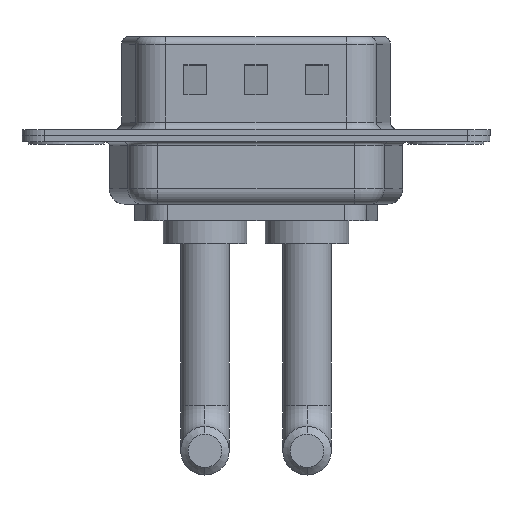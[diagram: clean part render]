
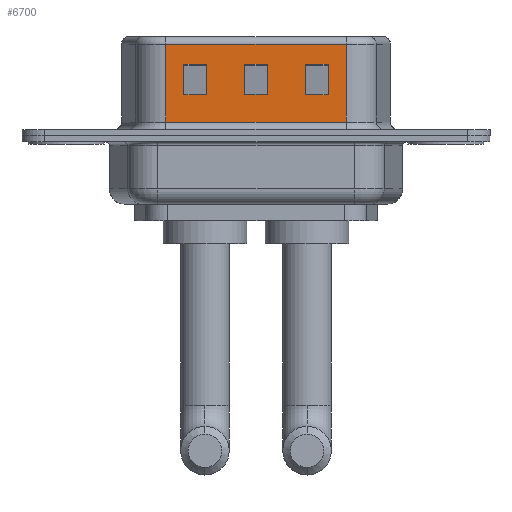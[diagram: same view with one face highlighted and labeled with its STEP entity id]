
A CAD part, front view. The second image highlights one B-rep face of the part: STEP entity #6700.
In plain terms, the highlighted planar face has unit normal (0, -1, 0).
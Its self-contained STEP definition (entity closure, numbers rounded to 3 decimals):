
#127 = EDGE_CURVE ( 'NONE', #7532, #10538, #2678, .T. ) ;
#140 = LINE ( 'NONE', #11574, #12310 ) ;
#228 = ORIENTED_EDGE ( 'NONE', *, *, #10622, .T. ) ;
#281 = DIRECTION ( 'NONE',  ( 0., 0., 1. ) ) ;
#351 = LINE ( 'NONE', #2179, #9631 ) ;
#443 = VERTEX_POINT ( 'NONE', #8490 ) ;
#605 = CARTESIAN_POINT ( 'NONE',  ( 18.451, -4.55, 0.9 ) ) ;
#623 = DIRECTION ( 'NONE',  ( 0., 1., 0. ) ) ;
#630 = CARTESIAN_POINT ( 'NONE',  ( 6.549, -4.55, 6.02 ) ) ;
#771 = ORIENTED_EDGE ( 'NONE', *, *, #10934, .F. ) ;
#1061 = ORIENTED_EDGE ( 'NONE', *, *, #8259, .T. ) ;
#1787 = EDGE_LOOP ( 'NONE', ( #228, #11066, #6406, #2359 ) ) ;
#1797 = FACE_BOUND ( 'NONE', #4188, .T. ) ;
#1937 = DIRECTION ( 'NONE',  ( 0., 0., -1. ) ) ;
#2086 = LINE ( 'NONE', #3164, #5693 ) ;
#2090 = CARTESIAN_POINT ( 'NONE',  ( 18.451, -4.55, 6.02 ) ) ;
#2119 = VECTOR ( 'NONE', #6483, 1000. ) ;
#2145 = DIRECTION ( 'NONE',  ( 1., 0., 0. ) ) ;
#2179 = CARTESIAN_POINT ( 'NONE',  ( 15.75, -4.55, 6.52 ) ) ;
#2353 = VERTEX_POINT ( 'NONE', #2929 ) ;
#2359 = ORIENTED_EDGE ( 'NONE', *, *, #7183, .T. ) ;
#2406 = LINE ( 'NONE', #5481, #9683 ) ;
#2586 = LINE ( 'NONE', #6353, #2119 ) ;
#2648 = EDGE_LOOP ( 'NONE', ( #1061, #12330, #9384, #11401 ) ) ;
#2678 = LINE ( 'NONE', #8633, #5533 ) ;
#2910 = DIRECTION ( 'NONE',  ( 1., 0., 0. ) ) ;
#2929 = CARTESIAN_POINT ( 'NONE',  ( 17.25, -4.55, 2.705 ) ) ;
#2930 = EDGE_CURVE ( 'NONE', #5158, #11398, #2086, .T. ) ;
#3065 = EDGE_CURVE ( 'NONE', #11744, #443, #2406, .T. ) ;
#3164 = CARTESIAN_POINT ( 'NONE',  ( 18.451, -4.55, 2.705 ) ) ;
#3402 = ORIENTED_EDGE ( 'NONE', *, *, #8332, .T. ) ;
#3432 = CARTESIAN_POINT ( 'NONE',  ( 18.451, -4.55, 6.52 ) ) ;
#3457 = VERTEX_POINT ( 'NONE', #6943 ) ;
#3461 = CARTESIAN_POINT ( 'NONE',  ( 15.75, -4.55, 4.705 ) ) ;
#3590 = CARTESIAN_POINT ( 'NONE',  ( 11.75, -4.55, 2.705 ) ) ;
#3946 = VECTOR ( 'NONE', #10274, 1000. ) ;
#4059 = DIRECTION ( 'NONE',  ( 0., 0., -1. ) ) ;
#4090 = EDGE_CURVE ( 'NONE', #2353, #8831, #5876, .T. ) ;
#4129 = DIRECTION ( 'NONE',  ( 1., 0., 0. ) ) ;
#4188 = EDGE_LOOP ( 'NONE', ( #3402, #8569, #7565, #4711 ) ) ;
#4375 = CARTESIAN_POINT ( 'NONE',  ( 18.451, -4.55, 4.705 ) ) ;
#4378 = VERTEX_POINT ( 'NONE', #6639 ) ;
#4633 = PLANE ( 'NONE',  #5189 ) ;
#4634 = VERTEX_POINT ( 'NONE', #10133 ) ;
#4681 = CARTESIAN_POINT ( 'NONE',  ( 9.25, -4.55, 6.52 ) ) ;
#4711 = ORIENTED_EDGE ( 'NONE', *, *, #9969, .T. ) ;
#4925 = CARTESIAN_POINT ( 'NONE',  ( 9.25, -4.55, 4.705 ) ) ;
#4926 = CARTESIAN_POINT ( 'NONE',  ( 22.451, -4.55, 2.705 ) ) ;
#5158 = VERTEX_POINT ( 'NONE', #11737 ) ;
#5166 = LINE ( 'NONE', #10057, #6983 ) ;
#5189 = AXIS2_PLACEMENT_3D ( 'NONE', #10415, #623, #7556 ) ;
#5291 = DIRECTION ( 'NONE',  ( 0., 0., 1. ) ) ;
#5481 = CARTESIAN_POINT ( 'NONE',  ( 7.75, -4.55, 6.52 ) ) ;
#5533 = VECTOR ( 'NONE', #10711, 1000. ) ;
#5651 = FACE_BOUND ( 'NONE', #1787, .T. ) ;
#5668 = DIRECTION ( 'NONE',  ( 0., 0., 1. ) ) ;
#5693 = VECTOR ( 'NONE', #10802, 1000. ) ;
#5702 = EDGE_CURVE ( 'NONE', #8831, #10414, #351, .T. ) ;
#5755 = VECTOR ( 'NONE', #7916, 1000. ) ;
#5876 = LINE ( 'NONE', #4926, #7566 ) ;
#5933 = CARTESIAN_POINT ( 'NONE',  ( 17.25, -4.55, 4.705 ) ) ;
#6199 = VERTEX_POINT ( 'NONE', #8041 ) ;
#6353 = CARTESIAN_POINT ( 'NONE',  ( 13.25, -4.55, 6.52 ) ) ;
#6406 = ORIENTED_EDGE ( 'NONE', *, *, #5702, .T. ) ;
#6483 = DIRECTION ( 'NONE',  ( 0., 0., -1. ) ) ;
#6567 = CARTESIAN_POINT ( 'NONE',  ( 15.75, -4.55, 2.705 ) ) ;
#6591 = VECTOR ( 'NONE', #5668, 1000. ) ;
#6613 = VECTOR ( 'NONE', #11154, 1000. ) ;
#6639 = CARTESIAN_POINT ( 'NONE',  ( 11.75, -4.55, 4.705 ) ) ;
#6663 = CARTESIAN_POINT ( 'NONE',  ( 17.25, -4.55, 6.52 ) ) ;
#6700 = ADVANCED_FACE ( 'NONE', ( #1797, #5651, #9586, #6711 ), #4633, .F. ) ;
#6711 = FACE_OUTER_BOUND ( 'NONE', #10720, .T. ) ;
#6894 = CARTESIAN_POINT ( 'NONE',  ( 22.451, -4.55, 4.705 ) ) ;
#6943 = CARTESIAN_POINT ( 'NONE',  ( 6.549, -4.55, 0.9 ) ) ;
#6983 = VECTOR ( 'NONE', #4129, 1000. ) ;
#7183 = EDGE_CURVE ( 'NONE', #10414, #7270, #8817, .T. ) ;
#7199 = VECTOR ( 'NONE', #11296, 1000. ) ;
#7270 = VERTEX_POINT ( 'NONE', #5933 ) ;
#7532 = VERTEX_POINT ( 'NONE', #2090 ) ;
#7556 = DIRECTION ( 'NONE',  ( -1., 0., 0. ) ) ;
#7565 = ORIENTED_EDGE ( 'NONE', *, *, #3065, .T. ) ;
#7566 = VECTOR ( 'NONE', #8823, 1000. ) ;
#7599 = VECTOR ( 'NONE', #2910, 1000. ) ;
#7916 = DIRECTION ( 'NONE',  ( 1., 0., 0. ) ) ;
#7946 = LINE ( 'NONE', #4375, #10563 ) ;
#8041 = CARTESIAN_POINT ( 'NONE',  ( 9.25, -4.55, 2.705 ) ) ;
#8066 = LINE ( 'NONE', #11929, #6613 ) ;
#8259 = EDGE_CURVE ( 'NONE', #4378, #4634, #7946, .T. ) ;
#8322 = CARTESIAN_POINT ( 'NONE',  ( 7.75, -4.55, 2.705 ) ) ;
#8332 = EDGE_CURVE ( 'NONE', #11998, #6199, #10349, .T. ) ;
#8434 = LINE ( 'NONE', #3432, #3946 ) ;
#8490 = CARTESIAN_POINT ( 'NONE',  ( 7.75, -4.55, 4.705 ) ) ;
#8538 = LINE ( 'NONE', #8599, #6591 ) ;
#8569 = ORIENTED_EDGE ( 'NONE', *, *, #10892, .T. ) ;
#8599 = CARTESIAN_POINT ( 'NONE',  ( 11.75, -4.55, 6.52 ) ) ;
#8633 = CARTESIAN_POINT ( 'NONE',  ( 18.451, -4.55, 6.02 ) ) ;
#8798 = VERTEX_POINT ( 'NONE', #605 ) ;
#8817 = LINE ( 'NONE', #6894, #5755 ) ;
#8823 = DIRECTION ( 'NONE',  ( -1., 0., 0. ) ) ;
#8831 = VERTEX_POINT ( 'NONE', #6567 ) ;
#9384 = ORIENTED_EDGE ( 'NONE', *, *, #2930, .T. ) ;
#9483 = LINE ( 'NONE', #6663, #11067 ) ;
#9586 = FACE_BOUND ( 'NONE', #2648, .T. ) ;
#9631 = VECTOR ( 'NONE', #281, 1000. ) ;
#9683 = VECTOR ( 'NONE', #5291, 1000. ) ;
#9752 = EDGE_CURVE ( 'NONE', #3457, #8798, #10691, .T. ) ;
#9966 = ORIENTED_EDGE ( 'NONE', *, *, #12376, .T. ) ;
#9969 = EDGE_CURVE ( 'NONE', #443, #11998, #5166, .T. ) ;
#10057 = CARTESIAN_POINT ( 'NONE',  ( 14.451, -4.55, 4.705 ) ) ;
#10133 = CARTESIAN_POINT ( 'NONE',  ( 13.25, -4.55, 4.705 ) ) ;
#10142 = ORIENTED_EDGE ( 'NONE', *, *, #127, .T. ) ;
#10176 = EDGE_CURVE ( 'NONE', #11398, #4378, #8538, .T. ) ;
#10274 = DIRECTION ( 'NONE',  ( 0., 0., -1. ) ) ;
#10349 = LINE ( 'NONE', #4681, #7199 ) ;
#10414 = VERTEX_POINT ( 'NONE', #3461 ) ;
#10415 = CARTESIAN_POINT ( 'NONE',  ( 18.451, -4.55, 6.52 ) ) ;
#10538 = VERTEX_POINT ( 'NONE', #630 ) ;
#10544 = EDGE_CURVE ( 'NONE', #4634, #5158, #2586, .T. ) ;
#10563 = VECTOR ( 'NONE', #2145, 1000. ) ;
#10622 = EDGE_CURVE ( 'NONE', #7270, #2353, #9483, .T. ) ;
#10691 = LINE ( 'NONE', #11701, #7599 ) ;
#10711 = DIRECTION ( 'NONE',  ( -1., 0., 0. ) ) ;
#10720 = EDGE_LOOP ( 'NONE', ( #771, #10142, #9966, #12350 ) ) ;
#10802 = DIRECTION ( 'NONE',  ( -1., 0., 0. ) ) ;
#10892 = EDGE_CURVE ( 'NONE', #6199, #11744, #8066, .T. ) ;
#10934 = EDGE_CURVE ( 'NONE', #7532, #8798, #8434, .T. ) ;
#11066 = ORIENTED_EDGE ( 'NONE', *, *, #4090, .T. ) ;
#11067 = VECTOR ( 'NONE', #1937, 1000. ) ;
#11154 = DIRECTION ( 'NONE',  ( -1., 0., 0. ) ) ;
#11296 = DIRECTION ( 'NONE',  ( 0., 0., -1. ) ) ;
#11398 = VERTEX_POINT ( 'NONE', #3590 ) ;
#11401 = ORIENTED_EDGE ( 'NONE', *, *, #10176, .T. ) ;
#11574 = CARTESIAN_POINT ( 'NONE',  ( 6.549, -4.55, 6.52 ) ) ;
#11701 = CARTESIAN_POINT ( 'NONE',  ( 18.451, -4.55, 0.9 ) ) ;
#11737 = CARTESIAN_POINT ( 'NONE',  ( 13.25, -4.55, 2.705 ) ) ;
#11744 = VERTEX_POINT ( 'NONE', #8322 ) ;
#11929 = CARTESIAN_POINT ( 'NONE',  ( 14.451, -4.55, 2.705 ) ) ;
#11998 = VERTEX_POINT ( 'NONE', #4925 ) ;
#12310 = VECTOR ( 'NONE', #4059, 1000. ) ;
#12330 = ORIENTED_EDGE ( 'NONE', *, *, #10544, .T. ) ;
#12350 = ORIENTED_EDGE ( 'NONE', *, *, #9752, .T. ) ;
#12376 = EDGE_CURVE ( 'NONE', #10538, #3457, #140, .T. ) ;
